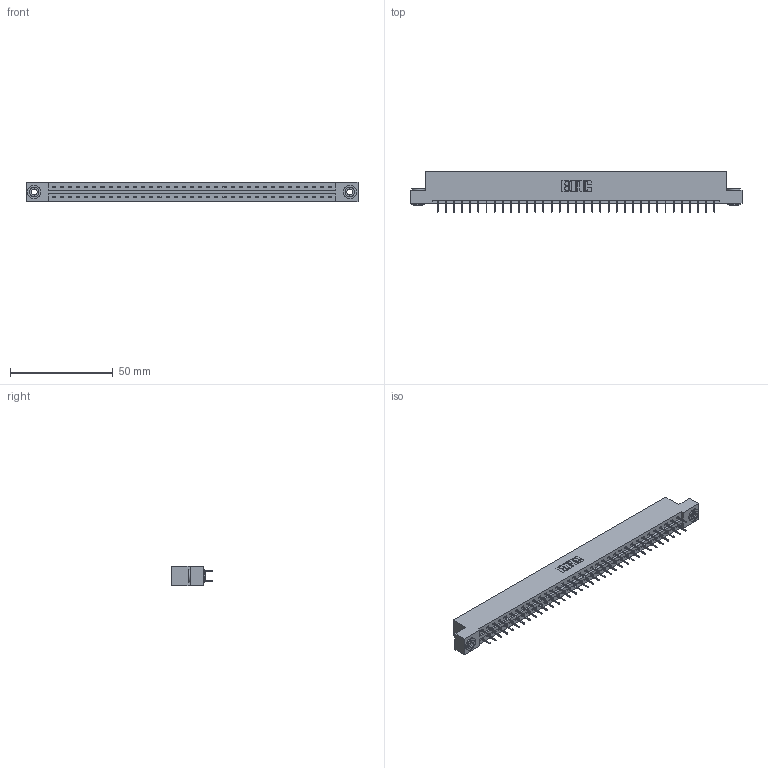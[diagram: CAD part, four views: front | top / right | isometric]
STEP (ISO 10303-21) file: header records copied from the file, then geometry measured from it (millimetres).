
FILE_DESCRIPTION (( 'STEP AP203' ), '1' );
FILE_NAME ('337-070-524-203.STEP', '2019-10-10T01:13:38', ( '' ), ( '' ), 'SwSTEP 2.0', 'SolidWorks 2016', '' );
FILE_SCHEMA (( 'CONFIG_CONTROL_DESIGN' ));
Length unit declared in the file: inch
Products named in the file (4): 337-070-524-203; 345-292-001_345-293-124; 337 Part_Flush Mounting Lugs - 0.156 Dia-TH; 345-250-002_345-250-002-102
Assembly tree (73 placements, depth 2):
  337-070-524-203
    337 Part_Flush Mounting Lugs - 0.156 Dia-TH
    345-292-001_345-293-124  x70
    345-250-002_345-250-002-102  x2
Bounding box: 161.7 x 19.69 x 9.4 mm (x, y, z)
Volume: 16861.1 mm3; surface area: 18889.9 mm2
Topology: 73 solids, 73 shells, 4212 faces, 11937 edges, 7674 vertices
Faces by surface type: plane 3160, cylinder 1044, cone 8
Entity records: 28766 total; most frequent: CARTESIAN_POINT 4825, ORIENTED_EDGE 4754, DIRECTION 4151, EDGE_CURVE 2377, VECTOR 2229, LINE 2229, VERTEX_POINT 1578, AXIS2_PLACEMENT_3D 961
